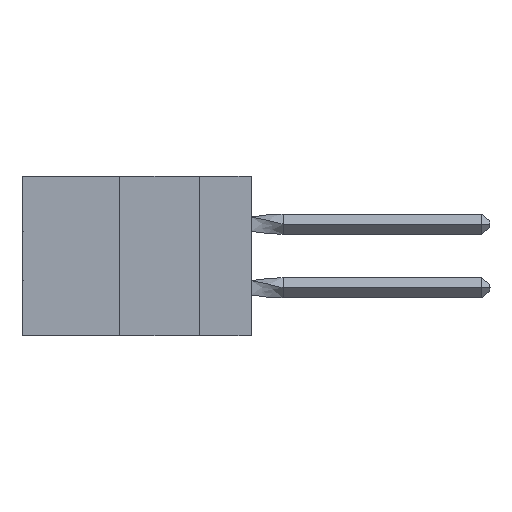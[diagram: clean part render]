
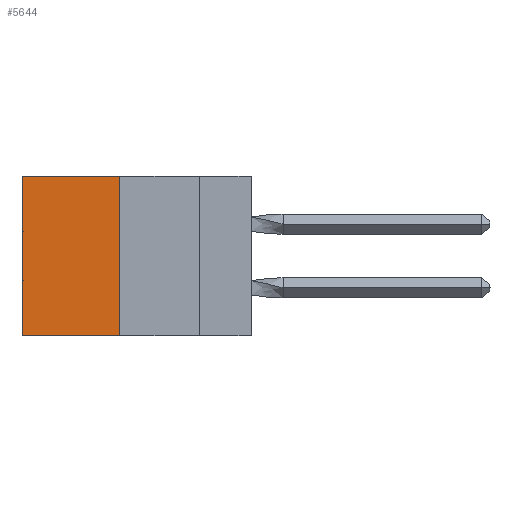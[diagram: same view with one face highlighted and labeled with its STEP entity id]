
A CAD part, left-side view. The second image highlights one B-rep face of the part: STEP entity #5644.
In plain terms, the highlighted planar face has unit normal (-1, 0, 0).
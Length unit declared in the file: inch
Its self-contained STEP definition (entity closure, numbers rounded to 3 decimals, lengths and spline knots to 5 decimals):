
#382 = CARTESIAN_POINT ( 'NONE',  ( 0.305, 0.413, 0. ) ) ;
#795 = CARTESIAN_POINT ( 'NONE',  ( 0.305, 0.72, -0.5 ) ) ;
#869 = CARTESIAN_POINT ( 'NONE',  ( 0.305, 0.413, -0.5 ) ) ;
#1061 = CARTESIAN_POINT ( 'NONE',  ( 0.305, 0.413, -0.5 ) ) ;
#1346 = VECTOR ( 'NONE', #36381, 39.37008 ) ;
#1698 = ORIENTED_EDGE ( 'NONE', *, *, #13822, .T. ) ;
#3580 = DIRECTION ( 'NONE',  ( 0., 1., 0. ) ) ;
#4887 = FACE_OUTER_BOUND ( 'NONE', #44424, .T. ) ;
#5605 = EDGE_CURVE ( 'NONE', #8003, #46401, #11840, .T. ) ;
#5644 = ADVANCED_FACE ( 'NONE', ( #4887 ), #24671, .F. ) ;
#6058 = ORIENTED_EDGE ( 'NONE', *, *, #17647, .T. ) ;
#6418 = VECTOR ( 'NONE', #19326, 39.37008 ) ;
#7752 = LINE ( 'NONE', #29102, #1346 ) ;
#8003 = VERTEX_POINT ( 'NONE', #34200 ) ;
#8305 = EDGE_CURVE ( 'NONE', #46401, #37062, #9903, .T. ) ;
#9903 = LINE ( 'NONE', #869, #6418 ) ;
#11840 = LINE ( 'NONE', #1061, #33630 ) ;
#13822 = EDGE_CURVE ( 'NONE', #31130, #37062, #7752, .T. ) ;
#14183 = VECTOR ( 'NONE', #3580, 39.37008 ) ;
#17647 = EDGE_CURVE ( 'NONE', #8003, #31130, #42299, .T. ) ;
#19326 = DIRECTION ( 'NONE',  ( 0., 1., 0. ) ) ;
#24671 = PLANE ( 'NONE',  #38366 ) ;
#28483 = DIRECTION ( 'NONE',  ( 0., 0., -1. ) ) ;
#29102 = CARTESIAN_POINT ( 'NONE',  ( 0.305, 0.72, -0.5 ) ) ;
#31130 = VERTEX_POINT ( 'NONE', #32641 ) ;
#32216 = ORIENTED_EDGE ( 'NONE', *, *, #8305, .F. ) ;
#32641 = CARTESIAN_POINT ( 'NONE',  ( 0.305, 0.72, 0. ) ) ;
#33630 = VECTOR ( 'NONE', #41547, 39.37008 ) ;
#34200 = CARTESIAN_POINT ( 'NONE',  ( 0.305, 0.413, 0. ) ) ;
#35585 = CARTESIAN_POINT ( 'NONE',  ( 0.305, 0.413, -0.5 ) ) ;
#35681 = ORIENTED_EDGE ( 'NONE', *, *, #5605, .F. ) ;
#36381 = DIRECTION ( 'NONE',  ( 0., 0., -1. ) ) ;
#37062 = VERTEX_POINT ( 'NONE', #795 ) ;
#37915 = CARTESIAN_POINT ( 'NONE',  ( 0.305, 0.413, -0.5 ) ) ;
#38366 = AXIS2_PLACEMENT_3D ( 'NONE', #35585, #42984, #28483 ) ;
#41547 = DIRECTION ( 'NONE',  ( 0., 0., -1. ) ) ;
#42299 = LINE ( 'NONE', #382, #14183 ) ;
#42984 = DIRECTION ( 'NONE',  ( 1., 0., 0. ) ) ;
#44424 = EDGE_LOOP ( 'NONE', ( #1698, #32216, #35681, #6058 ) ) ;
#46401 = VERTEX_POINT ( 'NONE', #37915 ) ;
